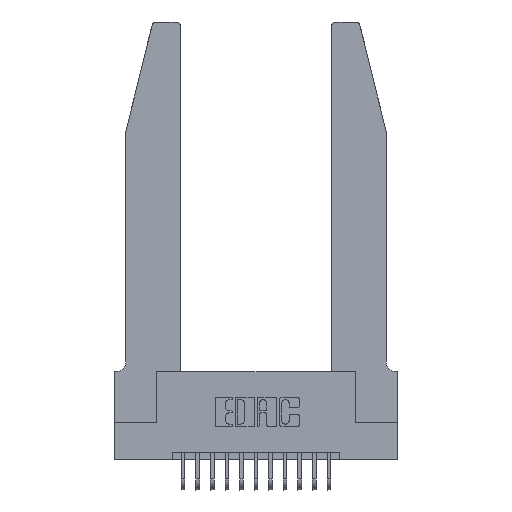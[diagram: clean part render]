
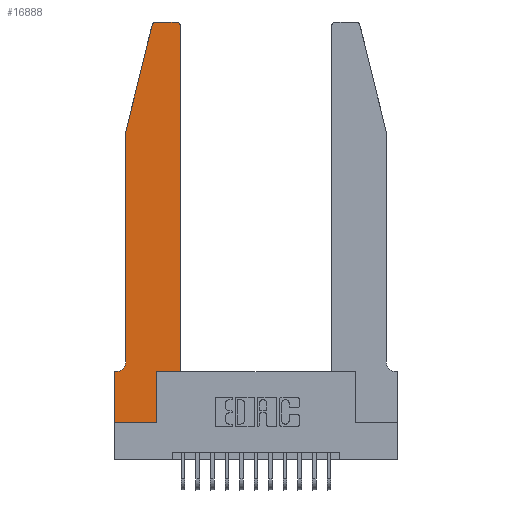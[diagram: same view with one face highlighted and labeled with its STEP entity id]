
A CAD part, top view. The second image highlights one B-rep face of the part: STEP entity #16888.
In plain terms, the highlighted planar face has unit normal (0, 0, 1).
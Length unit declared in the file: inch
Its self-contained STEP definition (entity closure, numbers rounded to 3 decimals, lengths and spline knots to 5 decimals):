
#241 = ORIENTED_EDGE ( 'NONE', *, *, #17255, .T. ) ;
#327 = ORIENTED_EDGE ( 'NONE', *, *, #11679, .T. ) ;
#460 = EDGE_CURVE ( 'NONE', #19011, #4355, #13744, .T. ) ;
#634 = VERTEX_POINT ( 'NONE', #10339 ) ;
#1147 = PLANE ( 'NONE',  #13415 ) ;
#1191 = LINE ( 'NONE', #18704, #4749 ) ;
#1326 = LINE ( 'NONE', #3997, #12309 ) ;
#1511 = CARTESIAN_POINT ( 'NONE',  ( 0., 0., 0.37 ) ) ;
#1737 = CARTESIAN_POINT ( 'NONE',  ( 0.4505, 2.72, 0.37 ) ) ;
#1748 = AXIS2_PLACEMENT_3D ( 'NONE', #5341, #15641, #6846 ) ;
#1757 = CARTESIAN_POINT ( 'NONE',  ( 0.2865, 0.35, 0.37 ) ) ;
#1773 = DIRECTION ( 'NONE',  ( -0.239, -0.971, 0. ) ) ;
#2263 = VERTEX_POINT ( 'NONE', #5787 ) ;
#2569 = EDGE_CURVE ( 'NONE', #4808, #6612, #1326, .T. ) ;
#2792 = CARTESIAN_POINT ( 'NONE',  ( 0., 0., 0.37 ) ) ;
#2868 = DIRECTION ( 'NONE',  ( 0., 1., 0. ) ) ;
#3283 = VECTOR ( 'NONE', #13087, 39.37008 ) ;
#3520 = CARTESIAN_POINT ( 'NONE',  ( 0.25487, 2.72718, 0.37 ) ) ;
#3745 = LINE ( 'NONE', #11618, #3283 ) ;
#3997 = CARTESIAN_POINT ( 'NONE',  ( 0., 0., 0.37 ) ) ;
#4021 = DIRECTION ( 'NONE',  ( 0., -1., 0. ) ) ;
#4147 = CARTESIAN_POINT ( 'NONE',  ( 0., 0.35, 0.37 ) ) ;
#4184 = EDGE_CURVE ( 'NONE', #5058, #11716, #14285, .T. ) ;
#4355 = VERTEX_POINT ( 'NONE', #6135 ) ;
#4529 = ORIENTED_EDGE ( 'NONE', *, *, #18036, .T. ) ;
#4697 = EDGE_CURVE ( 'NONE', #14476, #2263, #10417, .T. ) ;
#4749 = VECTOR ( 'NONE', #12911, 39.37008 ) ;
#4805 = CIRCLE ( 'NONE', #9623, 0.03 ) ;
#4808 = VERTEX_POINT ( 'NONE', #4147 ) ;
#5058 = VERTEX_POINT ( 'NONE', #12142 ) ;
#5081 = VECTOR ( 'NONE', #16403, 39.37008 ) ;
#5341 = CARTESIAN_POINT ( 'NONE',  ( 0.4205, 2.72, 0.37 ) ) ;
#5714 = DIRECTION ( 'NONE',  ( 1., 0., 0. ) ) ;
#5787 = CARTESIAN_POINT ( 'NONE',  ( 0.4205, 2.75, 0.37 ) ) ;
#5889 = VECTOR ( 'NONE', #1773, 39.37008 ) ;
#5955 = LINE ( 'NONE', #18416, #17222 ) ;
#6135 = CARTESIAN_POINT ( 'NONE',  ( 0.0755, 2., 0.37 ) ) ;
#6552 = ORIENTED_EDGE ( 'NONE', *, *, #460, .T. ) ;
#6612 = VERTEX_POINT ( 'NONE', #1511 ) ;
#6719 = EDGE_LOOP ( 'NONE', ( #327, #12611, #6552, #241, #8473, #4529, #13308, #9951, #14315, #17687, #12743, #11902 ) ) ;
#6846 = DIRECTION ( 'NONE',  ( 1., 0., 0. ) ) ;
#7312 = EDGE_CURVE ( 'NONE', #634, #9197, #16833, .T. ) ;
#7957 = VECTOR ( 'NONE', #11717, 39.37008 ) ;
#8473 = ORIENTED_EDGE ( 'NONE', *, *, #4184, .T. ) ;
#8760 = DIRECTION ( 'NONE',  ( 0., 0., -1. ) ) ;
#8786 = CARTESIAN_POINT ( 'NONE',  ( 0.0055, 0.35, 0.37 ) ) ;
#8891 = CARTESIAN_POINT ( 'NONE',  ( 0.284, 2.72, 0.37 ) ) ;
#9197 = VERTEX_POINT ( 'NONE', #1757 ) ;
#9623 = AXIS2_PLACEMENT_3D ( 'NONE', #8891, #19121, #10394 ) ;
#9758 = DIRECTION ( 'NONE',  ( 0., -1., 0. ) ) ;
#9951 = ORIENTED_EDGE ( 'NONE', *, *, #13132, .T. ) ;
#10339 = CARTESIAN_POINT ( 'NONE',  ( 0.2865, 0., 0.37 ) ) ;
#10394 = DIRECTION ( 'NONE',  ( 1., 0., 0. ) ) ;
#10417 = CIRCLE ( 'NONE', #1748, 0.03 ) ;
#11618 = CARTESIAN_POINT ( 'NONE',  ( 0.2605, 2.75, 0.37 ) ) ;
#11679 = EDGE_CURVE ( 'NONE', #2263, #12173, #3745, .T. ) ;
#11716 = VERTEX_POINT ( 'NONE', #8786 ) ;
#11717 = DIRECTION ( 'NONE',  ( 1., 0., 0. ) ) ;
#11902 = ORIENTED_EDGE ( 'NONE', *, *, #4697, .T. ) ;
#12087 = EDGE_CURVE ( 'NONE', #9197, #13240, #16255, .T. ) ;
#12142 = CARTESIAN_POINT ( 'NONE',  ( 0.0755, 0.42, 0.37 ) ) ;
#12173 = VERTEX_POINT ( 'NONE', #16900 ) ;
#12309 = VECTOR ( 'NONE', #4021, 39.37008 ) ;
#12436 = CARTESIAN_POINT ( 'NONE',  ( 0.4505, 0.35, 0.37 ) ) ;
#12611 = ORIENTED_EDGE ( 'NONE', *, *, #15916, .T. ) ;
#12675 = LINE ( 'NONE', #13257, #16576 ) ;
#12743 = ORIENTED_EDGE ( 'NONE', *, *, #15913, .T. ) ;
#12911 = DIRECTION ( 'NONE',  ( -1., 0., 0. ) ) ;
#13016 = CARTESIAN_POINT ( 'NONE',  ( 0., 0.35, 0.37 ) ) ;
#13087 = DIRECTION ( 'NONE',  ( -1., 0., 0. ) ) ;
#13132 = EDGE_CURVE ( 'NONE', #6612, #634, #14826, .T. ) ;
#13240 = VERTEX_POINT ( 'NONE', #17757 ) ;
#13257 = CARTESIAN_POINT ( 'NONE',  ( 0.4505, 0.35, 0.37 ) ) ;
#13308 = ORIENTED_EDGE ( 'NONE', *, *, #2569, .T. ) ;
#13415 = AXIS2_PLACEMENT_3D ( 'NONE', #13016, #14539, #5714 ) ;
#13462 = CARTESIAN_POINT ( 'NONE',  ( 0.2865, 0.35, 0.37 ) ) ;
#13744 = LINE ( 'NONE', #18039, #5889 ) ;
#14285 = CIRCLE ( 'NONE', #17362, 0.07 ) ;
#14315 = ORIENTED_EDGE ( 'NONE', *, *, #7312, .T. ) ;
#14476 = VERTEX_POINT ( 'NONE', #1737 ) ;
#14539 = DIRECTION ( 'NONE',  ( 0., 0., 1. ) ) ;
#14826 = LINE ( 'NONE', #2792, #7957 ) ;
#15395 = FACE_OUTER_BOUND ( 'NONE', #6719, .T. ) ;
#15641 = DIRECTION ( 'NONE',  ( 0., 0., 1. ) ) ;
#15778 = VECTOR ( 'NONE', #18284, 39.37008 ) ;
#15913 = EDGE_CURVE ( 'NONE', #13240, #14476, #12675, .T. ) ;
#15916 = EDGE_CURVE ( 'NONE', #12173, #19011, #4805, .T. ) ;
#16255 = LINE ( 'NONE', #12436, #15778 ) ;
#16403 = DIRECTION ( 'NONE',  ( 0., 1., 0. ) ) ;
#16576 = VECTOR ( 'NONE', #2868, 39.37008 ) ;
#16833 = LINE ( 'NONE', #13462, #5081 ) ;
#16888 = ADVANCED_FACE ( 'NONE', ( #15395 ), #1147, .T. ) ;
#16900 = CARTESIAN_POINT ( 'NONE',  ( 0.284, 2.75, 0.37 ) ) ;
#17222 = VECTOR ( 'NONE', #9758, 39.37008 ) ;
#17255 = EDGE_CURVE ( 'NONE', #4355, #5058, #5955, .T. ) ;
#17362 = AXIS2_PLACEMENT_3D ( 'NONE', #17515, #8760, #18986 ) ;
#17515 = CARTESIAN_POINT ( 'NONE',  ( 0.0055, 0.42, 0.37 ) ) ;
#17687 = ORIENTED_EDGE ( 'NONE', *, *, #12087, .T. ) ;
#17757 = CARTESIAN_POINT ( 'NONE',  ( 0.4505, 0.35, 0.37 ) ) ;
#18036 = EDGE_CURVE ( 'NONE', #11716, #4808, #1191, .T. ) ;
#18039 = CARTESIAN_POINT ( 'NONE',  ( 0.0755, 2., 0.37 ) ) ;
#18284 = DIRECTION ( 'NONE',  ( 1., 0., 0. ) ) ;
#18416 = CARTESIAN_POINT ( 'NONE',  ( 0.0755, 2., 0.37 ) ) ;
#18704 = CARTESIAN_POINT ( 'NONE',  ( 0.0755, 0.35, 0.37 ) ) ;
#18986 = DIRECTION ( 'NONE',  ( -1., 0., 0. ) ) ;
#19011 = VERTEX_POINT ( 'NONE', #3520 ) ;
#19121 = DIRECTION ( 'NONE',  ( 0., 0., 1. ) ) ;
